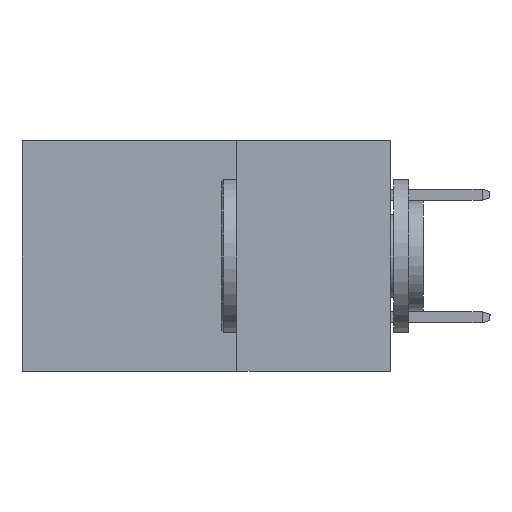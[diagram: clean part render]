
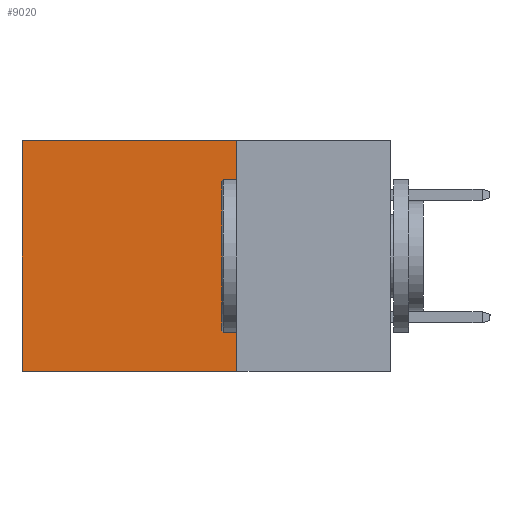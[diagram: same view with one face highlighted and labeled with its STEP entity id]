
A CAD part, left-side view. The second image highlights one B-rep face of the part: STEP entity #9020.
In plain terms, the highlighted planar face has unit normal (-1, 0, 0).
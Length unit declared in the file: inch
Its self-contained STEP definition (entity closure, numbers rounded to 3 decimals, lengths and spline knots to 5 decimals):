
#1712 = CARTESIAN_POINT ( 'NONE',  ( 0.2875, 0.25, -0.375 ) ) ;
#1758 = EDGE_CURVE ( 'NONE', #19143, #7094, #20669, .T. ) ;
#3497 = DIRECTION ( 'NONE',  ( 0., 1., 0. ) ) ;
#4636 = DIRECTION ( 'NONE',  ( 0., 1., 0. ) ) ;
#6411 = DIRECTION ( 'NONE',  ( 1., 0., 0. ) ) ;
#7085 = DIRECTION ( 'NONE',  ( 0., 0., -1. ) ) ;
#7094 = VERTEX_POINT ( 'NONE', #13542 ) ;
#7753 = ORIENTED_EDGE ( 'NONE', *, *, #14728, .T. ) ;
#7995 = CARTESIAN_POINT ( 'NONE',  ( 0.2875, 0.25, -0.375 ) ) ;
#8846 = VECTOR ( 'NONE', #7085, 39.37008 ) ;
#9020 = ADVANCED_FACE ( 'NONE', ( #10010 ), #16653, .F. ) ;
#9395 = LINE ( 'NONE', #19546, #8846 ) ;
#9682 = DIRECTION ( 'NONE',  ( 0., 0., -1. ) ) ;
#10010 = FACE_OUTER_BOUND ( 'NONE', #12360, .T. ) ;
#10366 = AXIS2_PLACEMENT_3D ( 'NONE', #15049, #6411, #9682 ) ;
#10703 = EDGE_CURVE ( 'NONE', #7094, #20533, #14870, .T. ) ;
#12360 = EDGE_LOOP ( 'NONE', ( #22176, #22365, #17133, #7753 ) ) ;
#13542 = CARTESIAN_POINT ( 'NONE',  ( 0.2875, 0.25, -0.375 ) ) ;
#14717 = VECTOR ( 'NONE', #4636, 39.37008 ) ;
#14728 = EDGE_CURVE ( 'NONE', #19143, #14915, #16628, .T. ) ;
#14870 = LINE ( 'NONE', #1712, #16224 ) ;
#14915 = VERTEX_POINT ( 'NONE', #17301 ) ;
#15049 = CARTESIAN_POINT ( 'NONE',  ( 0.2875, 0.25, -0.375 ) ) ;
#15413 = CARTESIAN_POINT ( 'NONE',  ( 0.2875, 0.6, -0.375 ) ) ;
#16224 = VECTOR ( 'NONE', #3497, 39.37008 ) ;
#16628 = LINE ( 'NONE', #18362, #14717 ) ;
#16653 = PLANE ( 'NONE',  #10366 ) ;
#16722 = DIRECTION ( 'NONE',  ( 0., 0., -1. ) ) ;
#17133 = ORIENTED_EDGE ( 'NONE', *, *, #1758, .F. ) ;
#17180 = EDGE_CURVE ( 'NONE', #14915, #20533, #9395, .T. ) ;
#17301 = CARTESIAN_POINT ( 'NONE',  ( 0.2875, 0.6, 0. ) ) ;
#18362 = CARTESIAN_POINT ( 'NONE',  ( 0.2875, 0.25, 0. ) ) ;
#19143 = VERTEX_POINT ( 'NONE', #21283 ) ;
#19546 = CARTESIAN_POINT ( 'NONE',  ( 0.2875, 0.6, -0.375 ) ) ;
#19582 = VECTOR ( 'NONE', #16722, 39.37008 ) ;
#20533 = VERTEX_POINT ( 'NONE', #15413 ) ;
#20669 = LINE ( 'NONE', #7995, #19582 ) ;
#21283 = CARTESIAN_POINT ( 'NONE',  ( 0.2875, 0.25, 0. ) ) ;
#22176 = ORIENTED_EDGE ( 'NONE', *, *, #17180, .T. ) ;
#22365 = ORIENTED_EDGE ( 'NONE', *, *, #10703, .F. ) ;
